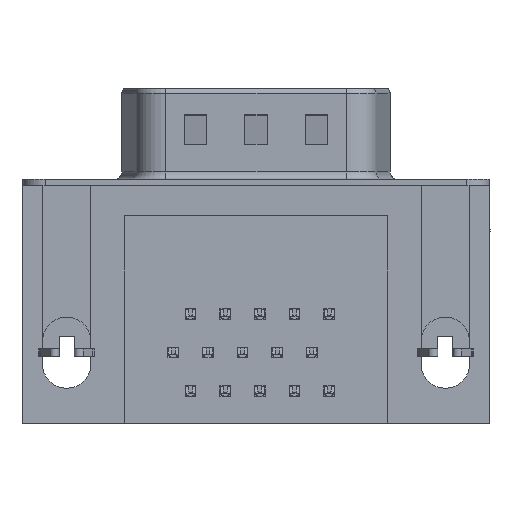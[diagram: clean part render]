
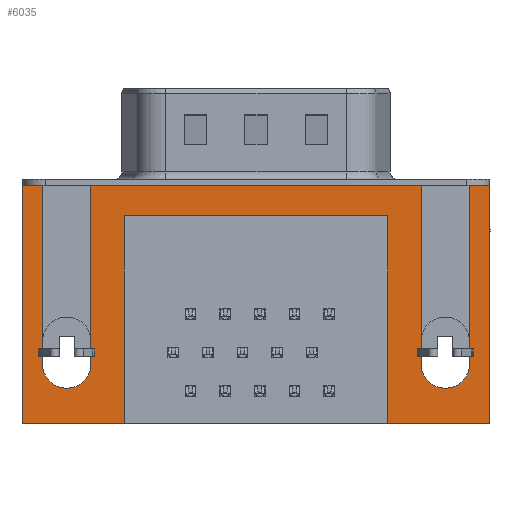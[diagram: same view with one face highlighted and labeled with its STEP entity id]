
A CAD part, front view. The second image highlights one B-rep face of the part: STEP entity #6035.
In plain terms, the highlighted planar face has unit normal (0, -1, 0).
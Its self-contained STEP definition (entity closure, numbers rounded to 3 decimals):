
#33 = VERTEX_POINT ( 'NONE', #11637 ) ;
#35 = CARTESIAN_POINT ( 'NONE',  ( -1.6, -6.275, -11.78 ) ) ;
#509 = AXIS2_PLACEMENT_3D ( 'NONE', #15721, #5375, #17468 ) ;
#659 = AXIS2_PLACEMENT_3D ( 'NONE', #11007, #746, #12745 ) ;
#667 = CIRCLE ( 'NONE', #659, 1.6 ) ;
#700 = ORIENTED_EDGE ( 'NONE', *, *, #10055, .F. ) ;
#733 = ORIENTED_EDGE ( 'NONE', *, *, #18063, .F. ) ;
#746 = DIRECTION ( 'NONE',  ( 0., -1., 0. ) ) ;
#942 = CARTESIAN_POINT ( 'NONE',  ( 3.79, -6.275, -15.7 ) ) ;
#1566 = VECTOR ( 'NONE', #13135, 1000. ) ;
#1807 = AXIS2_PLACEMENT_3D ( 'NONE', #3082, #15153, #4807 ) ;
#1960 = ORIENTED_EDGE ( 'NONE', *, *, #3390, .F. ) ;
#2128 = CARTESIAN_POINT ( 'NONE',  ( 0., -6.275, -13.38 ) ) ;
#2187 = VECTOR ( 'NONE', #9290, 1000. ) ;
#2293 = VERTEX_POINT ( 'NONE', #12216 ) ;
#2467 = ORIENTED_EDGE ( 'NONE', *, *, #7246, .F. ) ;
#2824 = CARTESIAN_POINT ( 'NONE',  ( -2.91, -6.275, 0. ) ) ;
#3082 = CARTESIAN_POINT ( 'NONE',  ( -2.91, -6.275, -2.5 ) ) ;
#3176 = VECTOR ( 'NONE', #9166, 1000. ) ;
#3182 = ORIENTED_EDGE ( 'NONE', *, *, #19465, .F. ) ;
#3390 = EDGE_CURVE ( 'NONE', #19792, #5809, #21262, .T. ) ;
#3500 = VERTEX_POINT ( 'NONE', #17024 ) ;
#3516 = DIRECTION ( 'NONE',  ( 0., 0., 1. ) ) ;
#3696 = EDGE_CURVE ( 'NONE', #16161, #12318, #16410, .T. ) ;
#3986 = CARTESIAN_POINT ( 'NONE',  ( 27.9, -6.275, -15.7 ) ) ;
#4058 = VECTOR ( 'NONE', #14306, 1000. ) ;
#4226 = DIRECTION ( 'NONE',  ( -1., 0., 0. ) ) ;
#4757 = LINE ( 'NONE', #17746, #9342 ) ;
#4807 = DIRECTION ( 'NONE',  ( 0., 0., -1. ) ) ;
#4880 = VERTEX_POINT ( 'NONE', #12414 ) ;
#5375 = DIRECTION ( 'NONE',  ( 0., -1., 0. ) ) ;
#5447 = CARTESIAN_POINT ( 'NONE',  ( 24.99, -6.275, -11.78 ) ) ;
#5757 = LINE ( 'NONE', #8556, #19545 ) ;
#5809 = VERTEX_POINT ( 'NONE', #7039 ) ;
#5994 = ORIENTED_EDGE ( 'NONE', *, *, #10991, .F. ) ;
#6035 = ADVANCED_FACE ( 'NONE', ( #16523 ), #11649, .T. ) ;
#6160 = VERTEX_POINT ( 'NONE', #35 ) ;
#6356 = CARTESIAN_POINT ( 'NONE',  ( -2.91, -6.275, -2.5 ) ) ;
#6386 = ORIENTED_EDGE ( 'NONE', *, *, #17115, .F. ) ;
#6625 = AXIS2_PLACEMENT_3D ( 'NONE', #5447, #17538, #7195 ) ;
#6766 = LINE ( 'NONE', #11002, #2187 ) ;
#6969 = ORIENTED_EDGE ( 'NONE', *, *, #17254, .F. ) ;
#7039 = CARTESIAN_POINT ( 'NONE',  ( 23.39, -6.275, 0. ) ) ;
#7076 = EDGE_CURVE ( 'NONE', #12247, #3500, #6766, .T. ) ;
#7103 = DIRECTION ( 'NONE',  ( -1., 0., 0. ) ) ;
#7195 = DIRECTION ( 'NONE',  ( 0., 0., 1. ) ) ;
#7246 = EDGE_CURVE ( 'NONE', #4880, #12247, #14059, .T. ) ;
#7470 = VERTEX_POINT ( 'NONE', #8688 ) ;
#7472 = VERTEX_POINT ( 'NONE', #20735 ) ;
#7502 = LINE ( 'NONE', #15703, #11493 ) ;
#7531 = VECTOR ( 'NONE', #18463, 1000. ) ;
#7857 = LINE ( 'NONE', #11845, #16482 ) ;
#7991 = VECTOR ( 'NONE', #11370, 1000. ) ;
#8293 = DIRECTION ( 'NONE',  ( 0., -1., 0. ) ) ;
#8556 = CARTESIAN_POINT ( 'NONE',  ( -1.6, -6.275, 0. ) ) ;
#8688 = CARTESIAN_POINT ( 'NONE',  ( 27.9, -6.275, 0. ) ) ;
#8844 = EDGE_CURVE ( 'NONE', #7472, #7470, #21542, .T. ) ;
#9166 = DIRECTION ( 'NONE',  ( 0., 0., 1. ) ) ;
#9290 = DIRECTION ( 'NONE',  ( 1., 0., 0. ) ) ;
#9342 = VECTOR ( 'NONE', #12501, 1000. ) ;
#9565 = EDGE_CURVE ( 'NONE', #11150, #2293, #20714, .T. ) ;
#9743 = DIRECTION ( 'NONE',  ( 0., 0., 1. ) ) ;
#9915 = ORIENTED_EDGE ( 'NONE', *, *, #3696, .F. ) ;
#9960 = VECTOR ( 'NONE', #13102, 1000. ) ;
#9995 = CARTESIAN_POINT ( 'NONE',  ( 26.59, -6.275, 0. ) ) ;
#10055 = EDGE_CURVE ( 'NONE', #7472, #16161, #7502, .T. ) ;
#10129 = VERTEX_POINT ( 'NONE', #2128 ) ;
#10991 = EDGE_CURVE ( 'NONE', #33, #13387, #17162, .T. ) ;
#11002 = CARTESIAN_POINT ( 'NONE',  ( -2.91, -6.275, 0. ) ) ;
#11007 = CARTESIAN_POINT ( 'NONE',  ( 24.99, -6.275, -11.78 ) ) ;
#11150 = VERTEX_POINT ( 'NONE', #15253 ) ;
#11266 = VECTOR ( 'NONE', #3516, 1000. ) ;
#11370 = DIRECTION ( 'NONE',  ( 0., 0., -1. ) ) ;
#11493 = VECTOR ( 'NONE', #7103, 1000. ) ;
#11637 = CARTESIAN_POINT ( 'NONE',  ( 3.79, -6.275, -2. ) ) ;
#11649 = PLANE ( 'NONE',  #1807 ) ;
#11769 = ORIENTED_EDGE ( 'NONE', *, *, #13216, .F. ) ;
#11845 = CARTESIAN_POINT ( 'NONE',  ( 23.39, -6.275, 0. ) ) ;
#12216 = CARTESIAN_POINT ( 'NONE',  ( 24.99, -6.275, -13.38 ) ) ;
#12235 = ORIENTED_EDGE ( 'NONE', *, *, #8844, .T. ) ;
#12247 = VERTEX_POINT ( 'NONE', #14979 ) ;
#12318 = VERTEX_POINT ( 'NONE', #20311 ) ;
#12335 = VERTEX_POINT ( 'NONE', #9995 ) ;
#12414 = CARTESIAN_POINT ( 'NONE',  ( -2.91, -6.275, -15.7 ) ) ;
#12501 = DIRECTION ( 'NONE',  ( 0., 0., 1. ) ) ;
#12685 = EDGE_CURVE ( 'NONE', #2293, #16020, #667, .T. ) ;
#12745 = DIRECTION ( 'NONE',  ( 0., 0., 1. ) ) ;
#12904 = CARTESIAN_POINT ( 'NONE',  ( 1.6, -6.275, 0. ) ) ;
#12915 = VERTEX_POINT ( 'NONE', #15036 ) ;
#13102 = DIRECTION ( 'NONE',  ( 0., 0., 1. ) ) ;
#13113 = CARTESIAN_POINT ( 'NONE',  ( 3.79, -6.275, -2. ) ) ;
#13135 = DIRECTION ( 'NONE',  ( 1., 0., 0. ) ) ;
#13212 = LINE ( 'NONE', #3986, #4058 ) ;
#13216 = EDGE_CURVE ( 'NONE', #12915, #19792, #4757, .T. ) ;
#13387 = VERTEX_POINT ( 'NONE', #942 ) ;
#13506 = VECTOR ( 'NONE', #9743, 1000. ) ;
#13527 = EDGE_LOOP ( 'NONE', ( #14334, #17600, #21366, #6386, #1960, #11769, #3182, #6969, #17305, #19959, #2467, #733, #5994, #13603, #9915, #700, #12235, #21079 ) ) ;
#13573 = DIRECTION ( 'NONE',  ( 0., 0., -1. ) ) ;
#13603 = ORIENTED_EDGE ( 'NONE', *, *, #18567, .F. ) ;
#13850 = CARTESIAN_POINT ( 'NONE',  ( 26.59, -6.275, -11.78 ) ) ;
#14059 = LINE ( 'NONE', #6356, #13506 ) ;
#14306 = DIRECTION ( 'NONE',  ( -1., 0., 0. ) ) ;
#14334 = ORIENTED_EDGE ( 'NONE', *, *, #18671, .F. ) ;
#14540 = LINE ( 'NONE', #19982, #9960 ) ;
#14762 = LINE ( 'NONE', #2824, #1566 ) ;
#14979 = CARTESIAN_POINT ( 'NONE',  ( -2.91, -6.275, 0. ) ) ;
#15036 = CARTESIAN_POINT ( 'NONE',  ( 1.6, -6.275, -11.78 ) ) ;
#15153 = DIRECTION ( 'NONE',  ( 0., -1., 0. ) ) ;
#15253 = CARTESIAN_POINT ( 'NONE',  ( 23.39, -6.275, -11.78 ) ) ;
#15496 = DIRECTION ( 'NONE',  ( 0., 0., -1. ) ) ;
#15597 = CARTESIAN_POINT ( 'NONE',  ( 27.9, -6.275, -2.5 ) ) ;
#15703 = CARTESIAN_POINT ( 'NONE',  ( 27.9, -6.275, -15.7 ) ) ;
#15721 = CARTESIAN_POINT ( 'NONE',  ( 0., -6.275, -11.78 ) ) ;
#16020 = VERTEX_POINT ( 'NONE', #13850 ) ;
#16161 = VERTEX_POINT ( 'NONE', #19458 ) ;
#16410 = LINE ( 'NONE', #21222, #3176 ) ;
#16482 = VECTOR ( 'NONE', #13573, 1000. ) ;
#16523 = FACE_OUTER_BOUND ( 'NONE', #13527, .T. ) ;
#16735 = CARTESIAN_POINT ( 'NONE',  ( -2.91, -6.275, 0. ) ) ;
#16737 = VECTOR ( 'NONE', #4226, 1000. ) ;
#17024 = CARTESIAN_POINT ( 'NONE',  ( -1.6, -6.275, 0. ) ) ;
#17111 = AXIS2_PLACEMENT_3D ( 'NONE', #18612, #8293, #20322 ) ;
#17115 = EDGE_CURVE ( 'NONE', #5809, #11150, #7857, .T. ) ;
#17162 = LINE ( 'NONE', #13113, #7991 ) ;
#17254 = EDGE_CURVE ( 'NONE', #6160, #10129, #18913, .T. ) ;
#17275 = LINE ( 'NONE', #17977, #16737 ) ;
#17305 = ORIENTED_EDGE ( 'NONE', *, *, #20762, .F. ) ;
#17468 = DIRECTION ( 'NONE',  ( 0., 0., -1. ) ) ;
#17538 = DIRECTION ( 'NONE',  ( 0., -1., 0. ) ) ;
#17600 = ORIENTED_EDGE ( 'NONE', *, *, #12685, .F. ) ;
#17746 = CARTESIAN_POINT ( 'NONE',  ( 1.6, -6.275, 0. ) ) ;
#17977 = CARTESIAN_POINT ( 'NONE',  ( 3.79, -6.275, -2. ) ) ;
#18063 = EDGE_CURVE ( 'NONE', #13387, #4880, #13212, .T. ) ;
#18463 = DIRECTION ( 'NONE',  ( 1., 0., 0. ) ) ;
#18567 = EDGE_CURVE ( 'NONE', #12318, #33, #17275, .T. ) ;
#18612 = CARTESIAN_POINT ( 'NONE',  ( 0., -6.275, -11.78 ) ) ;
#18671 = EDGE_CURVE ( 'NONE', #16020, #12335, #14540, .T. ) ;
#18851 = CIRCLE ( 'NONE', #17111, 1.6 ) ;
#18913 = CIRCLE ( 'NONE', #509, 1.6 ) ;
#19458 = CARTESIAN_POINT ( 'NONE',  ( 21.2, -6.275, -15.7 ) ) ;
#19465 = EDGE_CURVE ( 'NONE', #10129, #12915, #18851, .T. ) ;
#19545 = VECTOR ( 'NONE', #15496, 1000. ) ;
#19792 = VERTEX_POINT ( 'NONE', #12904 ) ;
#19901 = EDGE_CURVE ( 'NONE', #12335, #7470, #14762, .T. ) ;
#19959 = ORIENTED_EDGE ( 'NONE', *, *, #7076, .F. ) ;
#19982 = CARTESIAN_POINT ( 'NONE',  ( 26.59, -6.275, 0. ) ) ;
#20311 = CARTESIAN_POINT ( 'NONE',  ( 21.2, -6.275, -2. ) ) ;
#20322 = DIRECTION ( 'NONE',  ( 0., 0., -1. ) ) ;
#20714 = CIRCLE ( 'NONE', #6625, 1.6 ) ;
#20735 = CARTESIAN_POINT ( 'NONE',  ( 27.9, -6.275, -15.7 ) ) ;
#20762 = EDGE_CURVE ( 'NONE', #3500, #6160, #5757, .T. ) ;
#21079 = ORIENTED_EDGE ( 'NONE', *, *, #19901, .F. ) ;
#21222 = CARTESIAN_POINT ( 'NONE',  ( 21.2, -6.275, -2. ) ) ;
#21262 = LINE ( 'NONE', #16735, #7531 ) ;
#21366 = ORIENTED_EDGE ( 'NONE', *, *, #9565, .F. ) ;
#21542 = LINE ( 'NONE', #15597, #11266 ) ;
